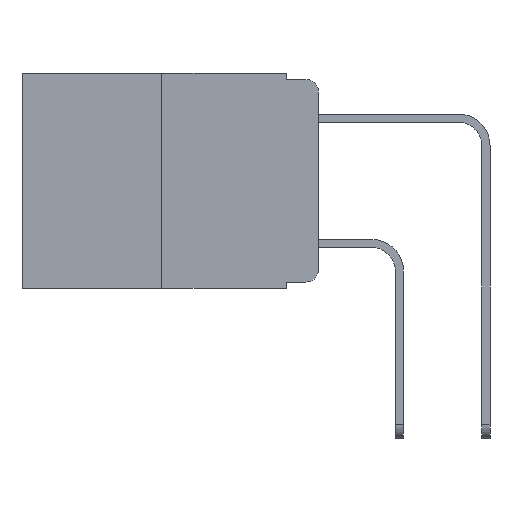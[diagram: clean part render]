
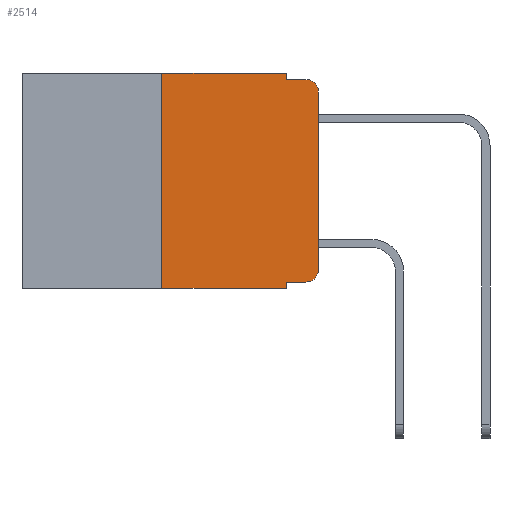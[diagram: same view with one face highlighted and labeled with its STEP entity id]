
A CAD part, left-side view. The second image highlights one B-rep face of the part: STEP entity #2514.
In plain terms, the highlighted planar face has unit normal (-1, 0, 0).
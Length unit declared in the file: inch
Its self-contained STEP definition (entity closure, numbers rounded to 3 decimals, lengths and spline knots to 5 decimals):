
#98 = AXIS2_PLACEMENT_3D ( 'NONE', #8398, #8598, #1893 ) ;
#482 = DIRECTION ( 'NONE',  ( 1., 0., 0. ) ) ;
#635 = VERTEX_POINT ( 'NONE', #7743 ) ;
#718 = VECTOR ( 'NONE', #2885, 39.37008 ) ;
#880 = DIRECTION ( 'NONE',  ( 0., 0., -1. ) ) ;
#886 = VERTEX_POINT ( 'NONE', #2130 ) ;
#1037 = LINE ( 'NONE', #8677, #718 ) ;
#1118 = CARTESIAN_POINT ( 'NONE',  ( 0., 0.473, 0. ) ) ;
#1173 = VECTOR ( 'NONE', #10320, 39.37008 ) ;
#1332 = VECTOR ( 'NONE', #4127, 39.37008 ) ;
#1500 = PLANE ( 'NONE',  #8700 ) ;
#1760 = ORIENTED_EDGE ( 'NONE', *, *, #11794, .T. ) ;
#1796 = ORIENTED_EDGE ( 'NONE', *, *, #3275, .F. ) ;
#1893 = DIRECTION ( 'NONE',  ( 0., 0., -1. ) ) ;
#2021 = VERTEX_POINT ( 'NONE', #11736 ) ;
#2130 = CARTESIAN_POINT ( 'NONE',  ( 0., 0.051, -0.333 ) ) ;
#2255 = DIRECTION ( 'NONE',  ( 0., -1., 0. ) ) ;
#2404 = VERTEX_POINT ( 'NONE', #9203 ) ;
#2493 = CARTESIAN_POINT ( 'NONE',  ( 0., 0.051, -0.01 ) ) ;
#2514 = ADVANCED_FACE ( 'NONE', ( #5204 ), #1500, .F. ) ;
#2630 = ORIENTED_EDGE ( 'NONE', *, *, #7664, .T. ) ;
#2857 = ORIENTED_EDGE ( 'NONE', *, *, #10603, .T. ) ;
#2885 = DIRECTION ( 'NONE',  ( 0., 0., 1. ) ) ;
#2886 = VERTEX_POINT ( 'NONE', #6084 ) ;
#3029 = VERTEX_POINT ( 'NONE', #6836 ) ;
#3275 = EDGE_CURVE ( 'NONE', #3029, #4035, #4626, .T. ) ;
#3510 = CIRCLE ( 'NONE', #98, 0.02 ) ;
#3514 = EDGE_CURVE ( 'NONE', #11043, #635, #3829, .T. ) ;
#3685 = EDGE_CURVE ( 'NONE', #886, #2404, #4921, .T. ) ;
#3829 = LINE ( 'NONE', #9081, #1173 ) ;
#3940 = CARTESIAN_POINT ( 'NONE',  ( 0., 0.02, -0.333 ) ) ;
#4035 = VERTEX_POINT ( 'NONE', #12035 ) ;
#4127 = DIRECTION ( 'NONE',  ( 0., -1., 0. ) ) ;
#4214 = VECTOR ( 'NONE', #2255, 39.37008 ) ;
#4287 = VECTOR ( 'NONE', #9253, 39.37008 ) ;
#4296 = VECTOR ( 'NONE', #4841, 39.37008 ) ;
#4626 = LINE ( 'NONE', #12193, #4296 ) ;
#4841 = DIRECTION ( 'NONE',  ( 0., 0., 1. ) ) ;
#4921 = LINE ( 'NONE', #9378, #4287 ) ;
#5168 = EDGE_CURVE ( 'NONE', #12217, #6486, #3510, .T. ) ;
#5204 = FACE_OUTER_BOUND ( 'NONE', #5556, .T. ) ;
#5212 = DIRECTION ( 'NONE',  ( 0., -1., 0. ) ) ;
#5248 = ORIENTED_EDGE ( 'NONE', *, *, #5168, .T. ) ;
#5442 = CARTESIAN_POINT ( 'NONE',  ( 0., 0.473, -0.343 ) ) ;
#5556 = EDGE_LOOP ( 'NONE', ( #2857, #8600, #10823, #8769, #8404, #1796, #2630, #8200, #1760, #5248 ) ) ;
#5737 = VECTOR ( 'NONE', #11164, 39.37008 ) ;
#5794 = CARTESIAN_POINT ( 'NONE',  ( 0., 0.051, 0. ) ) ;
#6084 = CARTESIAN_POINT ( 'NONE',  ( 0., 0.02, -0.01 ) ) ;
#6486 = VERTEX_POINT ( 'NONE', #10665 ) ;
#6836 = CARTESIAN_POINT ( 'NONE',  ( 0., 0.25, -0.343 ) ) ;
#6936 = CARTESIAN_POINT ( 'NONE',  ( 0., 0.02, -0.03 ) ) ;
#6954 = VECTOR ( 'NONE', #5212, 39.37008 ) ;
#6982 = EDGE_CURVE ( 'NONE', #4035, #11043, #8280, .T. ) ;
#7476 = EDGE_CURVE ( 'NONE', #635, #2886, #11634, .T. ) ;
#7522 = LINE ( 'NONE', #5442, #6954 ) ;
#7664 = EDGE_CURVE ( 'NONE', #3029, #2404, #7522, .T. ) ;
#7743 = CARTESIAN_POINT ( 'NONE',  ( 0., 0.051, -0.01 ) ) ;
#8200 = ORIENTED_EDGE ( 'NONE', *, *, #3685, .F. ) ;
#8280 = LINE ( 'NONE', #11178, #5737 ) ;
#8398 = CARTESIAN_POINT ( 'NONE',  ( 0., 0.02, -0.313 ) ) ;
#8404 = ORIENTED_EDGE ( 'NONE', *, *, #6982, .F. ) ;
#8598 = DIRECTION ( 'NONE',  ( -1., 0., 0. ) ) ;
#8600 = ORIENTED_EDGE ( 'NONE', *, *, #8969, .T. ) ;
#8677 = CARTESIAN_POINT ( 'NONE',  ( 0., 0., 0. ) ) ;
#8700 = AXIS2_PLACEMENT_3D ( 'NONE', #1118, #482, #880 ) ;
#8769 = ORIENTED_EDGE ( 'NONE', *, *, #3514, .F. ) ;
#8901 = CARTESIAN_POINT ( 'NONE',  ( 0., 0.051, -0.333 ) ) ;
#8969 = EDGE_CURVE ( 'NONE', #2021, #2886, #9376, .T. ) ;
#9081 = CARTESIAN_POINT ( 'NONE',  ( 0., 0.051, 0. ) ) ;
#9113 = AXIS2_PLACEMENT_3D ( 'NONE', #6936, #10599, #10559 ) ;
#9203 = CARTESIAN_POINT ( 'NONE',  ( 0., 0.051, -0.343 ) ) ;
#9253 = DIRECTION ( 'NONE',  ( 0., 0., -1. ) ) ;
#9376 = CIRCLE ( 'NONE', #9113, 0.02 ) ;
#9378 = CARTESIAN_POINT ( 'NONE',  ( 0., 0.051, 0. ) ) ;
#10320 = DIRECTION ( 'NONE',  ( 0., 0., -1. ) ) ;
#10559 = DIRECTION ( 'NONE',  ( 0., 0., -1. ) ) ;
#10599 = DIRECTION ( 'NONE',  ( -1., 0., 0. ) ) ;
#10603 = EDGE_CURVE ( 'NONE', #6486, #2021, #1037, .T. ) ;
#10665 = CARTESIAN_POINT ( 'NONE',  ( 0., 0., -0.313 ) ) ;
#10823 = ORIENTED_EDGE ( 'NONE', *, *, #7476, .F. ) ;
#11043 = VERTEX_POINT ( 'NONE', #5794 ) ;
#11164 = DIRECTION ( 'NONE',  ( 0., -1., 0. ) ) ;
#11178 = CARTESIAN_POINT ( 'NONE',  ( 0., 0.473, 0. ) ) ;
#11429 = LINE ( 'NONE', #8901, #1332 ) ;
#11634 = LINE ( 'NONE', #2493, #4214 ) ;
#11736 = CARTESIAN_POINT ( 'NONE',  ( 0., 0., -0.03 ) ) ;
#11794 = EDGE_CURVE ( 'NONE', #886, #12217, #11429, .T. ) ;
#12035 = CARTESIAN_POINT ( 'NONE',  ( 0., 0.25, 0. ) ) ;
#12193 = CARTESIAN_POINT ( 'NONE',  ( 0., 0.25, 0. ) ) ;
#12217 = VERTEX_POINT ( 'NONE', #3940 ) ;
